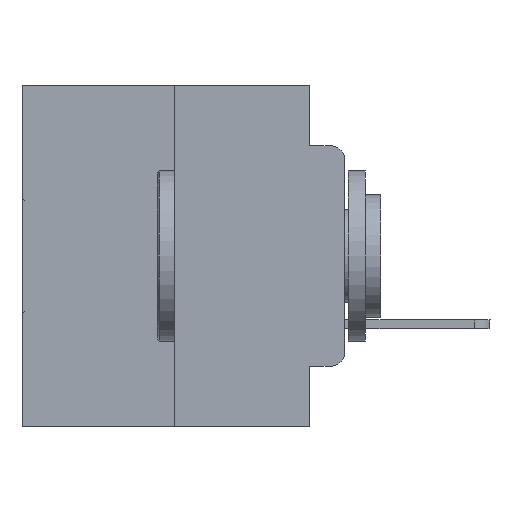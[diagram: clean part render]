
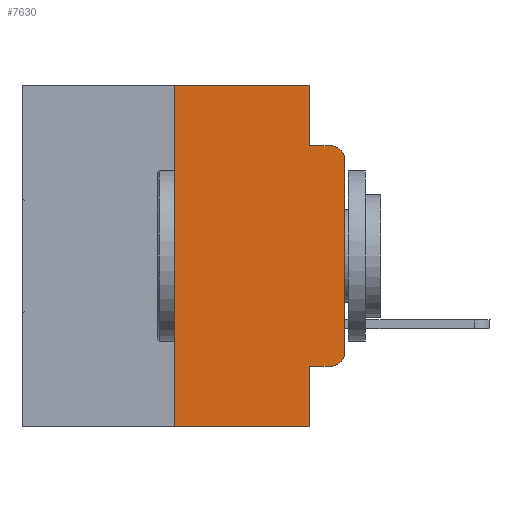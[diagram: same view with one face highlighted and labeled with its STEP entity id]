
A CAD part, left-side view. The second image highlights one B-rep face of the part: STEP entity #7630.
In plain terms, the highlighted planar face has unit normal (-1, 0, 0).
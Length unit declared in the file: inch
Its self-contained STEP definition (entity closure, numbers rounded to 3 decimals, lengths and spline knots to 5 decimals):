
#56 = EDGE_CURVE ( 'NONE', #23304, #4158, #27108, .T. ) ;
#80 = EDGE_CURVE ( 'NONE', #417, #13715, #19555, .T. ) ;
#417 = VERTEX_POINT ( 'NONE', #26930 ) ;
#504 = EDGE_CURVE ( 'NONE', #13905, #23304, #10586, .T. ) ;
#524 = DIRECTION ( 'NONE',  ( 0., 0., -1. ) ) ;
#545 = VERTEX_POINT ( 'NONE', #6051 ) ;
#1291 = CARTESIAN_POINT ( 'NONE',  ( 0., 0.02, -0.3915 ) ) ;
#1400 = CARTESIAN_POINT ( 'NONE',  ( 0., 0.051, 0. ) ) ;
#1709 = LINE ( 'NONE', #3233, #27570 ) ;
#2193 = EDGE_CURVE ( 'NONE', #13715, #10003, #7823, .T. ) ;
#2609 = CARTESIAN_POINT ( 'NONE',  ( 0., 0.25, -0.5 ) ) ;
#2805 = ORIENTED_EDGE ( 'NONE', *, *, #23950, .F. ) ;
#3143 = DIRECTION ( 'NONE',  ( 0., 0., 1. ) ) ;
#3233 = CARTESIAN_POINT ( 'NONE',  ( 0., 0.051, -0.4115 ) ) ;
#3290 = DIRECTION ( 'NONE',  ( 1., 0., 0. ) ) ;
#4158 = VERTEX_POINT ( 'NONE', #1400 ) ;
#5062 = LINE ( 'NONE', #13992, #12416 ) ;
#5128 = CARTESIAN_POINT ( 'NONE',  ( 0., 0.02, -0.1085 ) ) ;
#5332 = VERTEX_POINT ( 'NONE', #21919 ) ;
#5533 = DIRECTION ( 'NONE',  ( -1., 0., 0. ) ) ;
#5758 = DIRECTION ( 'NONE',  ( 0., 0., 1. ) ) ;
#5829 = AXIS2_PLACEMENT_3D ( 'NONE', #16219, #3290, #16648 ) ;
#6051 = CARTESIAN_POINT ( 'NONE',  ( 0., 0.051, -0.0885 ) ) ;
#6757 = CIRCLE ( 'NONE', #27790, 0.02 ) ;
#7182 = DIRECTION ( 'NONE',  ( -1., 0., 0. ) ) ;
#7253 = EDGE_CURVE ( 'NONE', #10003, #28646, #6757, .T. ) ;
#7264 = LINE ( 'NONE', #23248, #19090 ) ;
#7476 = DIRECTION ( 'NONE',  ( 0., 0., -1. ) ) ;
#7630 = ADVANCED_FACE ( 'NONE', ( #21189 ), #25435, .F. ) ;
#7641 = ORIENTED_EDGE ( 'NONE', *, *, #11275, .F. ) ;
#7823 = LINE ( 'NONE', #26010, #18162 ) ;
#8300 = VECTOR ( 'NONE', #9066, 39.37008 ) ;
#9066 = DIRECTION ( 'NONE',  ( 0., -1., 0. ) ) ;
#9729 = ORIENTED_EDGE ( 'NONE', *, *, #56, .F. ) ;
#10003 = VERTEX_POINT ( 'NONE', #13591 ) ;
#10586 = LINE ( 'NONE', #16925, #20971 ) ;
#10797 = DIRECTION ( 'NONE',  ( 0., -1., 0. ) ) ;
#11145 = AXIS2_PLACEMENT_3D ( 'NONE', #1291, #5533, #28112 ) ;
#11262 = ORIENTED_EDGE ( 'NONE', *, *, #2193, .T. ) ;
#11275 = EDGE_CURVE ( 'NONE', #5332, #19998, #19482, .T. ) ;
#11558 = CARTESIAN_POINT ( 'NONE',  ( 0., 0.051, -0.0885 ) ) ;
#11710 = CARTESIAN_POINT ( 'NONE',  ( 0., 0.473, 0. ) ) ;
#11849 = ORIENTED_EDGE ( 'NONE', *, *, #80, .T. ) ;
#11980 = VECTOR ( 'NONE', #18319, 39.37008 ) ;
#12416 = VECTOR ( 'NONE', #22973, 39.37008 ) ;
#12440 = CARTESIAN_POINT ( 'NONE',  ( 0., 0., -0.3915 ) ) ;
#13591 = CARTESIAN_POINT ( 'NONE',  ( 0., 0., -0.1085 ) ) ;
#13715 = VERTEX_POINT ( 'NONE', #12440 ) ;
#13739 = LINE ( 'NONE', #11558, #11980 ) ;
#13905 = VERTEX_POINT ( 'NONE', #2609 ) ;
#13992 = CARTESIAN_POINT ( 'NONE',  ( 0., 0.473, -0.5 ) ) ;
#14071 = CARTESIAN_POINT ( 'NONE',  ( 0., 0.02, -0.0885 ) ) ;
#14783 = CARTESIAN_POINT ( 'NONE',  ( 0., 0.25, 0. ) ) ;
#16219 = CARTESIAN_POINT ( 'NONE',  ( 0., 0.473, 0. ) ) ;
#16648 = DIRECTION ( 'NONE',  ( 0., 0., -1. ) ) ;
#16925 = CARTESIAN_POINT ( 'NONE',  ( 0., 0.25, 0. ) ) ;
#17178 = ORIENTED_EDGE ( 'NONE', *, *, #25067, .T. ) ;
#18162 = VECTOR ( 'NONE', #3143, 39.37008 ) ;
#18319 = DIRECTION ( 'NONE',  ( 0., -1., 0. ) ) ;
#19090 = VECTOR ( 'NONE', #524, 39.37008 ) ;
#19482 = LINE ( 'NONE', #28540, #27097 ) ;
#19555 = CIRCLE ( 'NONE', #11145, 0.02 ) ;
#19998 = VERTEX_POINT ( 'NONE', #26345 ) ;
#20144 = EDGE_CURVE ( 'NONE', #13905, #19998, #5062, .T. ) ;
#20558 = ORIENTED_EDGE ( 'NONE', *, *, #504, .F. ) ;
#20971 = VECTOR ( 'NONE', #5758, 39.37008 ) ;
#21045 = EDGE_CURVE ( 'NONE', #545, #28646, #13739, .T. ) ;
#21081 = ORIENTED_EDGE ( 'NONE', *, *, #7253, .T. ) ;
#21086 = ORIENTED_EDGE ( 'NONE', *, *, #20144, .T. ) ;
#21189 = FACE_OUTER_BOUND ( 'NONE', #21423, .T. ) ;
#21423 = EDGE_LOOP ( 'NONE', ( #11262, #21081, #22597, #2805, #9729, #20558, #21086, #7641, #17178, #11849 ) ) ;
#21919 = CARTESIAN_POINT ( 'NONE',  ( 0., 0.051, -0.4115 ) ) ;
#22597 = ORIENTED_EDGE ( 'NONE', *, *, #21045, .F. ) ;
#22973 = DIRECTION ( 'NONE',  ( 0., -1., 0. ) ) ;
#23248 = CARTESIAN_POINT ( 'NONE',  ( 0., 0.051, 0. ) ) ;
#23304 = VERTEX_POINT ( 'NONE', #14783 ) ;
#23950 = EDGE_CURVE ( 'NONE', #4158, #545, #7264, .T. ) ;
#25067 = EDGE_CURVE ( 'NONE', #5332, #417, #1709, .T. ) ;
#25435 = PLANE ( 'NONE',  #5829 ) ;
#26010 = CARTESIAN_POINT ( 'NONE',  ( 0., 0., 0. ) ) ;
#26345 = CARTESIAN_POINT ( 'NONE',  ( 0., 0.051, -0.5 ) ) ;
#26930 = CARTESIAN_POINT ( 'NONE',  ( 0., 0.02, -0.4115 ) ) ;
#27097 = VECTOR ( 'NONE', #28395, 39.37008 ) ;
#27108 = LINE ( 'NONE', #11710, #8300 ) ;
#27570 = VECTOR ( 'NONE', #10797, 39.37008 ) ;
#27790 = AXIS2_PLACEMENT_3D ( 'NONE', #5128, #7182, #7476 ) ;
#28112 = DIRECTION ( 'NONE',  ( 0., 0., -1. ) ) ;
#28395 = DIRECTION ( 'NONE',  ( 0., 0., -1. ) ) ;
#28540 = CARTESIAN_POINT ( 'NONE',  ( 0., 0.051, 0. ) ) ;
#28646 = VERTEX_POINT ( 'NONE', #14071 ) ;
